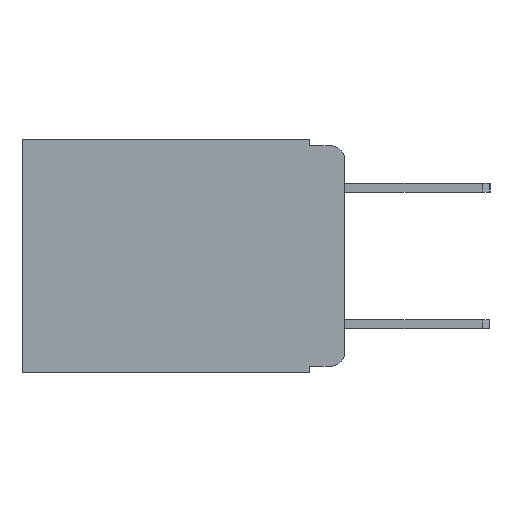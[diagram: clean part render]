
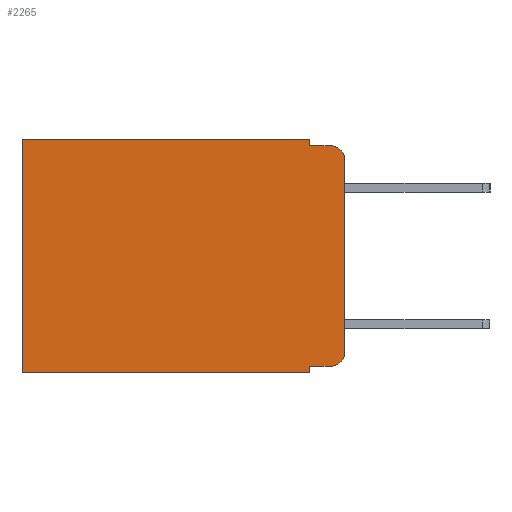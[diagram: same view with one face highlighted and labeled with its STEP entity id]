
A CAD part, left-side view. The second image highlights one B-rep face of the part: STEP entity #2265.
In plain terms, the highlighted planar face has unit normal (-1, 0, 0).
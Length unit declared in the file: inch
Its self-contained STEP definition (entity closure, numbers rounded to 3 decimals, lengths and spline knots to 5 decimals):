
#374 = VERTEX_POINT ( 'NONE', #7529 ) ;
#496 = EDGE_CURVE ( 'NONE', #10715, #374, #7187, .T. ) ;
#515 = CARTESIAN_POINT ( 'NONE',  ( 0.298, 0.051, -0.01 ) ) ;
#609 = DIRECTION ( 'NONE',  ( 0., 0., -1. ) ) ;
#830 = CARTESIAN_POINT ( 'NONE',  ( 0.298, 0.051, 0. ) ) ;
#876 = EDGE_CURVE ( 'NONE', #7189, #6870, #15175, .T. ) ;
#1220 = CARTESIAN_POINT ( 'NONE',  ( 0.298, 0., -0.313 ) ) ;
#1555 = VECTOR ( 'NONE', #9767, 39.37008 ) ;
#2094 = DIRECTION ( 'NONE',  ( 0., 0., -1. ) ) ;
#2231 = ORIENTED_EDGE ( 'NONE', *, *, #496, .T. ) ;
#2239 = LINE ( 'NONE', #830, #13795 ) ;
#2265 = ADVANCED_FACE ( 'NONE', ( #6582 ), #7981, .F. ) ;
#2375 = CARTESIAN_POINT ( 'NONE',  ( 0.298, 0.051, -0.343 ) ) ;
#2540 = DIRECTION ( 'NONE',  ( 0., 1., 0. ) ) ;
#2560 = EDGE_CURVE ( 'NONE', #7189, #2746, #12089, .T. ) ;
#2746 = VERTEX_POINT ( 'NONE', #1220 ) ;
#2779 = EDGE_LOOP ( 'NONE', ( #5356, #7418, #5134, #8257, #2231, #5856, #9306, #11939, #12288, #9656 ) ) ;
#2864 = VECTOR ( 'NONE', #11704, 39.37008 ) ;
#2932 = VERTEX_POINT ( 'NONE', #12273 ) ;
#3253 = LINE ( 'NONE', #7147, #2864 ) ;
#3414 = CARTESIAN_POINT ( 'NONE',  ( 0.298, 0.02, -0.01 ) ) ;
#3609 = DIRECTION ( 'NONE',  ( 0., 1., 0. ) ) ;
#3659 = EDGE_CURVE ( 'NONE', #2932, #2746, #13255, .T. ) ;
#3665 = DIRECTION ( 'NONE',  ( 0., -1., 0. ) ) ;
#3766 = CARTESIAN_POINT ( 'NONE',  ( 0.298, 0.473, -0.343 ) ) ;
#3843 = CARTESIAN_POINT ( 'NONE',  ( 0.298, 0.051, 0. ) ) ;
#4858 = LINE ( 'NONE', #3843, #1555 ) ;
#5134 = ORIENTED_EDGE ( 'NONE', *, *, #12955, .F. ) ;
#5342 = EDGE_CURVE ( 'NONE', #8287, #2932, #9291, .T. ) ;
#5356 = ORIENTED_EDGE ( 'NONE', *, *, #2560, .F. ) ;
#5386 = CARTESIAN_POINT ( 'NONE',  ( 0.298, 0., -0.343 ) ) ;
#5741 = AXIS2_PLACEMENT_3D ( 'NONE', #6295, #6415, #5951 ) ;
#5856 = ORIENTED_EDGE ( 'NONE', *, *, #10772, .T. ) ;
#5951 = DIRECTION ( 'NONE',  ( 0., 0., -1. ) ) ;
#6295 = CARTESIAN_POINT ( 'NONE',  ( 0.298, 0.02, -0.03 ) ) ;
#6415 = DIRECTION ( 'NONE',  ( -1., 0., 0. ) ) ;
#6582 = FACE_OUTER_BOUND ( 'NONE', #2779, .T. ) ;
#6612 = EDGE_CURVE ( 'NONE', #13345, #10878, #12403, .T. ) ;
#6870 = VERTEX_POINT ( 'NONE', #3414 ) ;
#7147 = CARTESIAN_POINT ( 'NONE',  ( 0.298, 0.473, 0. ) ) ;
#7187 = LINE ( 'NONE', #8276, #9544 ) ;
#7189 = VERTEX_POINT ( 'NONE', #12567 ) ;
#7418 = ORIENTED_EDGE ( 'NONE', *, *, #876, .T. ) ;
#7529 = CARTESIAN_POINT ( 'NONE',  ( 0.298, 0.473, 0. ) ) ;
#7852 = DIRECTION ( 'NONE',  ( 0., -1., 0. ) ) ;
#7911 = CARTESIAN_POINT ( 'NONE',  ( 0.298, 0., 0. ) ) ;
#7939 = DIRECTION ( 'NONE',  ( 0., 0., -1. ) ) ;
#7960 = DIRECTION ( 'NONE',  ( 1., 0., 0. ) ) ;
#7981 = PLANE ( 'NONE',  #12453 ) ;
#8046 = VECTOR ( 'NONE', #7852, 39.37008 ) ;
#8257 = ORIENTED_EDGE ( 'NONE', *, *, #11477, .F. ) ;
#8276 = CARTESIAN_POINT ( 'NONE',  ( 0.298, 0., 0. ) ) ;
#8287 = VERTEX_POINT ( 'NONE', #15049 ) ;
#8463 = EDGE_CURVE ( 'NONE', #8287, #13345, #4858, .T. ) ;
#8775 = VECTOR ( 'NONE', #12425, 39.37008 ) ;
#9157 = CARTESIAN_POINT ( 'NONE',  ( 0.298, 0.051, -0.01 ) ) ;
#9291 = LINE ( 'NONE', #10725, #9642 ) ;
#9306 = ORIENTED_EDGE ( 'NONE', *, *, #6612, .F. ) ;
#9423 = VECTOR ( 'NONE', #2540, 39.37008 ) ;
#9544 = VECTOR ( 'NONE', #3609, 39.37008 ) ;
#9642 = VECTOR ( 'NONE', #3665, 39.37008 ) ;
#9656 = ORIENTED_EDGE ( 'NONE', *, *, #3659, .T. ) ;
#9767 = DIRECTION ( 'NONE',  ( 0., 0., -1. ) ) ;
#10222 = DIRECTION ( 'NONE',  ( -1., 0., 0. ) ) ;
#10715 = VERTEX_POINT ( 'NONE', #11650 ) ;
#10725 = CARTESIAN_POINT ( 'NONE',  ( 0.298, 0.051, -0.333 ) ) ;
#10772 = EDGE_CURVE ( 'NONE', #374, #10878, #3253, .T. ) ;
#10878 = VERTEX_POINT ( 'NONE', #3766 ) ;
#11107 = AXIS2_PLACEMENT_3D ( 'NONE', #12757, #10222, #609 ) ;
#11477 = EDGE_CURVE ( 'NONE', #10715, #12240, #2239, .T. ) ;
#11615 = CARTESIAN_POINT ( 'NONE',  ( 0.298, 0., 0. ) ) ;
#11650 = CARTESIAN_POINT ( 'NONE',  ( 0.298, 0.051, 0. ) ) ;
#11704 = DIRECTION ( 'NONE',  ( 0., 0., -1. ) ) ;
#11939 = ORIENTED_EDGE ( 'NONE', *, *, #8463, .F. ) ;
#12089 = LINE ( 'NONE', #11615, #8775 ) ;
#12240 = VERTEX_POINT ( 'NONE', #9157 ) ;
#12273 = CARTESIAN_POINT ( 'NONE',  ( 0.298, 0.02, -0.333 ) ) ;
#12288 = ORIENTED_EDGE ( 'NONE', *, *, #5342, .T. ) ;
#12403 = LINE ( 'NONE', #5386, #9423 ) ;
#12425 = DIRECTION ( 'NONE',  ( 0., 0., -1. ) ) ;
#12453 = AXIS2_PLACEMENT_3D ( 'NONE', #7911, #7960, #7939 ) ;
#12567 = CARTESIAN_POINT ( 'NONE',  ( 0.298, 0., -0.03 ) ) ;
#12757 = CARTESIAN_POINT ( 'NONE',  ( 0.298, 0.02, -0.313 ) ) ;
#12955 = EDGE_CURVE ( 'NONE', #12240, #6870, #13270, .T. ) ;
#13255 = CIRCLE ( 'NONE', #11107, 0.02 ) ;
#13270 = LINE ( 'NONE', #515, #8046 ) ;
#13345 = VERTEX_POINT ( 'NONE', #2375 ) ;
#13795 = VECTOR ( 'NONE', #2094, 39.37008 ) ;
#15049 = CARTESIAN_POINT ( 'NONE',  ( 0.298, 0.051, -0.333 ) ) ;
#15175 = CIRCLE ( 'NONE', #5741, 0.02 ) ;
